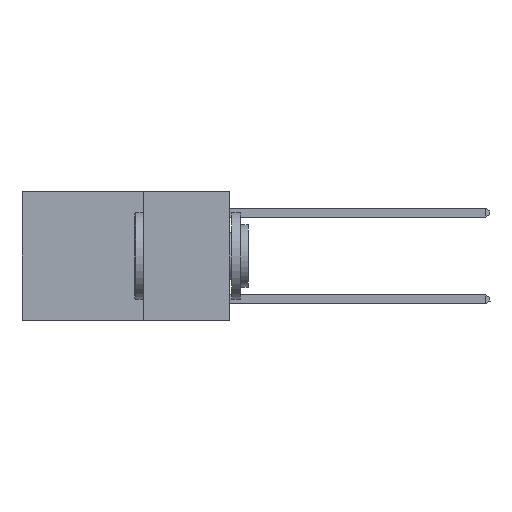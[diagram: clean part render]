
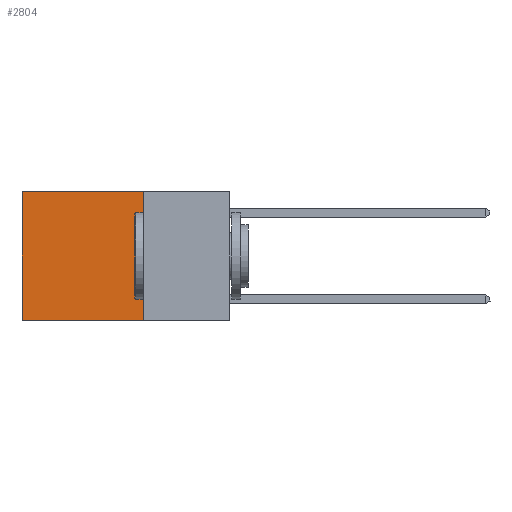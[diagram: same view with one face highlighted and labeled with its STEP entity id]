
A CAD part, left-side view. The second image highlights one B-rep face of the part: STEP entity #2804.
In plain terms, the highlighted planar face has unit normal (-1, 0, 0).
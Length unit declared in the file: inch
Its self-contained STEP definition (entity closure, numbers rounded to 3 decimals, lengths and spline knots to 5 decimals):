
#562 = CARTESIAN_POINT ( 'NONE',  ( 0.2625, 0.25, 0. ) ) ;
#1197 = CARTESIAN_POINT ( 'NONE',  ( 0.2625, 0.6, 0. ) ) ;
#2305 = DIRECTION ( 'NONE',  ( 0., 1., 0. ) ) ;
#2346 = EDGE_CURVE ( 'NONE', #16789, #14163, #7184, .T. ) ;
#2606 = CARTESIAN_POINT ( 'NONE',  ( 0.2625, 0.25, 0. ) ) ;
#2804 = ADVANCED_FACE ( 'NONE', ( #7459 ), #21532, .F. ) ;
#3063 = DIRECTION ( 'NONE',  ( 1., 0., 0. ) ) ;
#4595 = EDGE_CURVE ( 'NONE', #11533, #13730, #15542, .T. ) ;
#5244 = CARTESIAN_POINT ( 'NONE',  ( 0.2625, 0.6, 0. ) ) ;
#5460 = AXIS2_PLACEMENT_3D ( 'NONE', #16560, #3063, #14912 ) ;
#6056 = VECTOR ( 'NONE', #2305, 39.37008 ) ;
#6203 = DIRECTION ( 'NONE',  ( 0., 1., 0. ) ) ;
#6876 = ORIENTED_EDGE ( 'NONE', *, *, #11736, .T. ) ;
#7155 = EDGE_LOOP ( 'NONE', ( #6876, #19685, #21139, #17484 ) ) ;
#7184 = LINE ( 'NONE', #16296, #20018 ) ;
#7459 = FACE_OUTER_BOUND ( 'NONE', #7155, .T. ) ;
#8069 = CARTESIAN_POINT ( 'NONE',  ( 0.2625, 0.6, -0.37 ) ) ;
#10128 = VECTOR ( 'NONE', #14489, 39.37008 ) ;
#10398 = EDGE_CURVE ( 'NONE', #11533, #16789, #19004, .T. ) ;
#11097 = LINE ( 'NONE', #1197, #19457 ) ;
#11533 = VERTEX_POINT ( 'NONE', #19328 ) ;
#11736 = EDGE_CURVE ( 'NONE', #13730, #14163, #11097, .T. ) ;
#11804 = CARTESIAN_POINT ( 'NONE',  ( 0.2625, 0.25, -0.37 ) ) ;
#13121 = DIRECTION ( 'NONE',  ( 0., 0., -1. ) ) ;
#13730 = VERTEX_POINT ( 'NONE', #5244 ) ;
#14163 = VERTEX_POINT ( 'NONE', #8069 ) ;
#14489 = DIRECTION ( 'NONE',  ( 0., 0., -1. ) ) ;
#14912 = DIRECTION ( 'NONE',  ( 0., 0., -1. ) ) ;
#15542 = LINE ( 'NONE', #562, #6056 ) ;
#16296 = CARTESIAN_POINT ( 'NONE',  ( 0.2625, 0.25, -0.37 ) ) ;
#16560 = CARTESIAN_POINT ( 'NONE',  ( 0.2625, 0.25, 0. ) ) ;
#16789 = VERTEX_POINT ( 'NONE', #11804 ) ;
#17484 = ORIENTED_EDGE ( 'NONE', *, *, #4595, .T. ) ;
#19004 = LINE ( 'NONE', #2606, #10128 ) ;
#19328 = CARTESIAN_POINT ( 'NONE',  ( 0.2625, 0.25, 0. ) ) ;
#19457 = VECTOR ( 'NONE', #13121, 39.37008 ) ;
#19685 = ORIENTED_EDGE ( 'NONE', *, *, #2346, .F. ) ;
#20018 = VECTOR ( 'NONE', #6203, 39.37008 ) ;
#21139 = ORIENTED_EDGE ( 'NONE', *, *, #10398, .F. ) ;
#21532 = PLANE ( 'NONE',  #5460 ) ;
